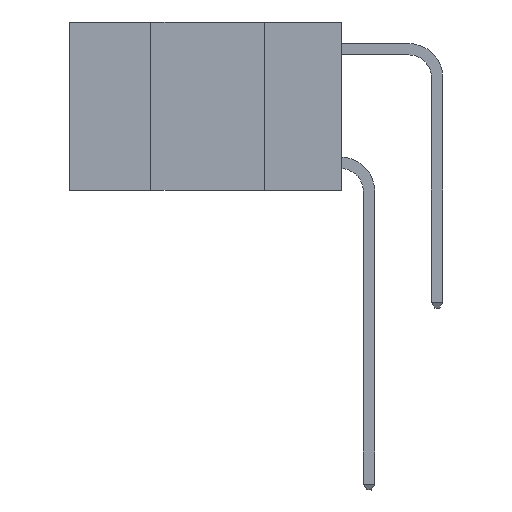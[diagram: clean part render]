
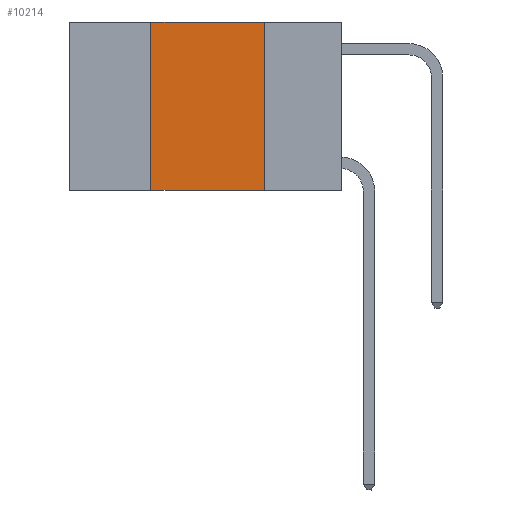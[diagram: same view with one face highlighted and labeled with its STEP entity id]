
A CAD part, left-side view. The second image highlights one B-rep face of the part: STEP entity #10214.
In plain terms, the highlighted planar face has unit normal (-1, 0, 0).
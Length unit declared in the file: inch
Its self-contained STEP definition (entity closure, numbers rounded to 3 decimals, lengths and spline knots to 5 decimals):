
#239 = CARTESIAN_POINT ( 'NONE',  ( 0., 0.42, -0.37 ) ) ;
#281 = VERTEX_POINT ( 'NONE', #3380 ) ;
#799 = ORIENTED_EDGE ( 'NONE', *, *, #4533, .F. ) ;
#1080 = DIRECTION ( 'NONE',  ( 0., 0., -1. ) ) ;
#1916 = CARTESIAN_POINT ( 'NONE',  ( 0., 0.6, 0. ) ) ;
#1935 = VERTEX_POINT ( 'NONE', #239 ) ;
#2042 = EDGE_CURVE ( 'NONE', #281, #9190, #6060, .T. ) ;
#2143 = VECTOR ( 'NONE', #7727, 39.37008 ) ;
#2281 = DIRECTION ( 'NONE',  ( 0., 0., 1. ) ) ;
#2293 = CARTESIAN_POINT ( 'NONE',  ( 0., 0.17, 0. ) ) ;
#2312 = VECTOR ( 'NONE', #2281, 39.37008 ) ;
#2527 = EDGE_CURVE ( 'NONE', #1935, #5778, #7858, .T. ) ;
#2739 = FACE_OUTER_BOUND ( 'NONE', #8278, .T. ) ;
#3143 = VECTOR ( 'NONE', #8308, 39.37008 ) ;
#3380 = CARTESIAN_POINT ( 'NONE',  ( 0., 0.42, 0. ) ) ;
#4533 = EDGE_CURVE ( 'NONE', #1935, #281, #7142, .T. ) ;
#4924 = DIRECTION ( 'NONE',  ( 0., 0., -1. ) ) ;
#5015 = CARTESIAN_POINT ( 'NONE',  ( 0., 0.6, -0.37 ) ) ;
#5237 = PLANE ( 'NONE',  #10491 ) ;
#5522 = CARTESIAN_POINT ( 'NONE',  ( 0., 0.17, -0.37 ) ) ;
#5778 = VERTEX_POINT ( 'NONE', #5522 ) ;
#6060 = LINE ( 'NONE', #1916, #2143 ) ;
#6087 = ORIENTED_EDGE ( 'NONE', *, *, #2042, .F. ) ;
#6511 = LINE ( 'NONE', #10649, #9253 ) ;
#7142 = LINE ( 'NONE', #8020, #2312 ) ;
#7228 = ORIENTED_EDGE ( 'NONE', *, *, #2527, .T. ) ;
#7702 = CARTESIAN_POINT ( 'NONE',  ( 0., 0.6, 0. ) ) ;
#7727 = DIRECTION ( 'NONE',  ( 0., -1., 0. ) ) ;
#7858 = LINE ( 'NONE', #5015, #3143 ) ;
#8020 = CARTESIAN_POINT ( 'NONE',  ( 0., 0.42, 0. ) ) ;
#8278 = EDGE_LOOP ( 'NONE', ( #10141, #6087, #799, #7228 ) ) ;
#8308 = DIRECTION ( 'NONE',  ( 0., -1., 0. ) ) ;
#9190 = VERTEX_POINT ( 'NONE', #2293 ) ;
#9253 = VECTOR ( 'NONE', #4924, 39.37008 ) ;
#9313 = DIRECTION ( 'NONE',  ( 1., 0., 0. ) ) ;
#9661 = EDGE_CURVE ( 'NONE', #9190, #5778, #6511, .T. ) ;
#10141 = ORIENTED_EDGE ( 'NONE', *, *, #9661, .F. ) ;
#10214 = ADVANCED_FACE ( 'NONE', ( #2739 ), #5237, .F. ) ;
#10491 = AXIS2_PLACEMENT_3D ( 'NONE', #7702, #9313, #1080 ) ;
#10649 = CARTESIAN_POINT ( 'NONE',  ( 0., 0.17, 0. ) ) ;
